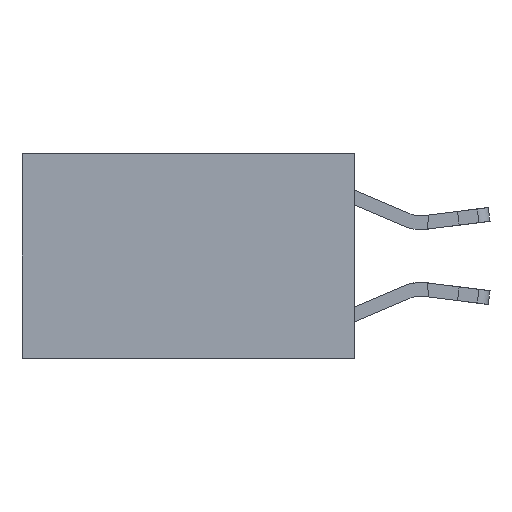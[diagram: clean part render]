
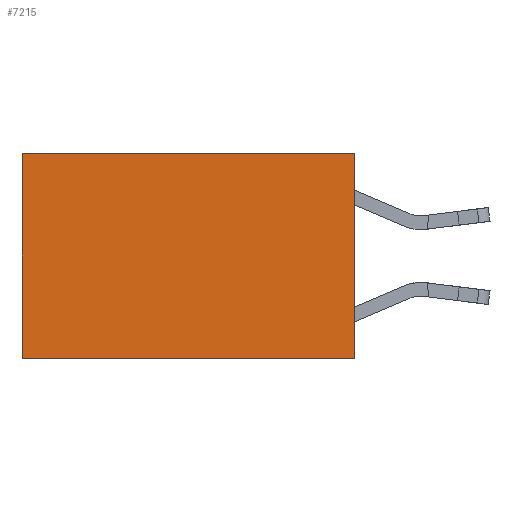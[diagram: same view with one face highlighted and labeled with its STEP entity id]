
A CAD part, left-side view. The second image highlights one B-rep face of the part: STEP entity #7215.
In plain terms, the highlighted planar face has unit normal (-1, 0, 0).
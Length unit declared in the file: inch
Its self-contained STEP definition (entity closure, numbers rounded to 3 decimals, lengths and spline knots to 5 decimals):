
#2329 = CARTESIAN_POINT ( 'NONE',  ( 0.2625, 0., 0. ) ) ;
#2871 = VECTOR ( 'NONE', #4090, 39.37008 ) ;
#3817 = DIRECTION ( 'NONE',  ( 0., 1., 0. ) ) ;
#4090 = DIRECTION ( 'NONE',  ( 0., 0., -1. ) ) ;
#4244 = LINE ( 'NONE', #12527, #8568 ) ;
#4508 = EDGE_CURVE ( 'NONE', #8860, #10887, #4244, .T. ) ;
#5507 = PLANE ( 'NONE',  #8215 ) ;
#6400 = ORIENTED_EDGE ( 'NONE', *, *, #11056, .F. ) ;
#6840 = LINE ( 'NONE', #11653, #2871 ) ;
#7215 = ADVANCED_FACE ( 'NONE', ( #16629 ), #5507, .F. ) ;
#7394 = ORIENTED_EDGE ( 'NONE', *, *, #4508, .T. ) ;
#7655 = VECTOR ( 'NONE', #7995, 39.37008 ) ;
#7995 = DIRECTION ( 'NONE',  ( 0., 1., 0. ) ) ;
#8215 = AXIS2_PLACEMENT_3D ( 'NONE', #2329, #20059, #9000 ) ;
#8568 = VECTOR ( 'NONE', #10667, 39.37008 ) ;
#8860 = VERTEX_POINT ( 'NONE', #16643 ) ;
#9000 = DIRECTION ( 'NONE',  ( 0., 0., -1. ) ) ;
#10064 = VECTOR ( 'NONE', #3817, 39.37008 ) ;
#10667 = DIRECTION ( 'NONE',  ( 0., 0., -1. ) ) ;
#10877 = VERTEX_POINT ( 'NONE', #16165 ) ;
#10887 = VERTEX_POINT ( 'NONE', #17446 ) ;
#11056 = EDGE_CURVE ( 'NONE', #10877, #16500, #6840, .T. ) ;
#11653 = CARTESIAN_POINT ( 'NONE',  ( 0.2625, 0., 0. ) ) ;
#12502 = LINE ( 'NONE', #12815, #7655 ) ;
#12527 = CARTESIAN_POINT ( 'NONE',  ( 0.2625, 0.6, 0. ) ) ;
#12815 = CARTESIAN_POINT ( 'NONE',  ( 0.2625, 0., -0.37 ) ) ;
#15141 = CARTESIAN_POINT ( 'NONE',  ( 0.2625, 0., 0. ) ) ;
#15750 = CARTESIAN_POINT ( 'NONE',  ( 0.2625, 0., -0.37 ) ) ;
#16165 = CARTESIAN_POINT ( 'NONE',  ( 0.2625, 0., 0. ) ) ;
#16500 = VERTEX_POINT ( 'NONE', #15750 ) ;
#16629 = FACE_OUTER_BOUND ( 'NONE', #18437, .T. ) ;
#16643 = CARTESIAN_POINT ( 'NONE',  ( 0.2625, 0.6, 0. ) ) ;
#17446 = CARTESIAN_POINT ( 'NONE',  ( 0.2625, 0.6, -0.37 ) ) ;
#18243 = ORIENTED_EDGE ( 'NONE', *, *, #20403, .T. ) ;
#18437 = EDGE_LOOP ( 'NONE', ( #7394, #19372, #6400, #18243 ) ) ;
#19372 = ORIENTED_EDGE ( 'NONE', *, *, #19646, .F. ) ;
#19646 = EDGE_CURVE ( 'NONE', #16500, #10887, #12502, .T. ) ;
#20059 = DIRECTION ( 'NONE',  ( 1., 0., 0. ) ) ;
#20403 = EDGE_CURVE ( 'NONE', #10877, #8860, #20608, .T. ) ;
#20608 = LINE ( 'NONE', #15141, #10064 ) ;
